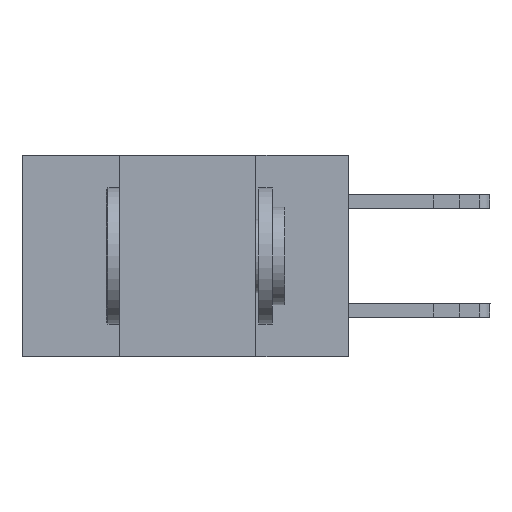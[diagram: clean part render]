
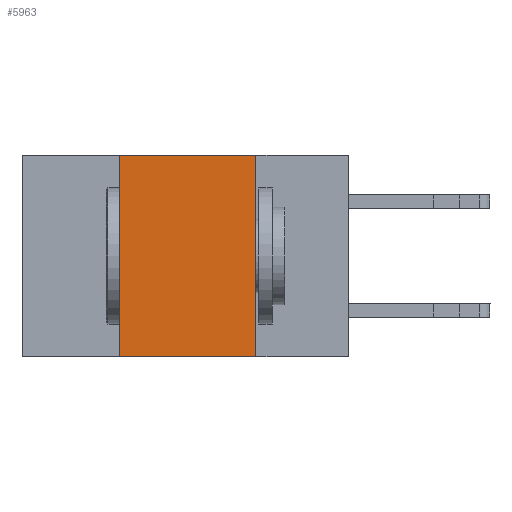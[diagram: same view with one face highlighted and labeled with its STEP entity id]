
A CAD part, left-side view. The second image highlights one B-rep face of the part: STEP entity #5963.
In plain terms, the highlighted planar face has unit normal (-1, 0, 0).
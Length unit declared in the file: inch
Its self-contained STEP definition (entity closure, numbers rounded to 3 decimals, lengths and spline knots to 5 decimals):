
#101 = ORIENTED_EDGE ( 'NONE', *, *, #4121, .F. ) ;
#929 = DIRECTION ( 'NONE',  ( 0., -1., 0. ) ) ;
#1136 = VERTEX_POINT ( 'NONE', #2300 ) ;
#1154 = VECTOR ( 'NONE', #8800, 39.37008 ) ;
#1475 = CARTESIAN_POINT ( 'NONE',  ( 0., 0.17, 0. ) ) ;
#1583 = LINE ( 'NONE', #4087, #10183 ) ;
#1917 = EDGE_CURVE ( 'NONE', #1136, #8242, #1583, .T. ) ;
#1934 = LINE ( 'NONE', #7120, #1154 ) ;
#2142 = DIRECTION ( 'NONE',  ( 0., 0., -1. ) ) ;
#2300 = CARTESIAN_POINT ( 'NONE',  ( 0., 0.42, -0.37 ) ) ;
#3206 = DIRECTION ( 'NONE',  ( 0., -1., 0. ) ) ;
#3469 = AXIS2_PLACEMENT_3D ( 'NONE', #3813, #5595, #2142 ) ;
#3813 = CARTESIAN_POINT ( 'NONE',  ( 0., 0.6, 0. ) ) ;
#3879 = PLANE ( 'NONE',  #3469 ) ;
#3974 = CARTESIAN_POINT ( 'NONE',  ( 0., 0.6, 0. ) ) ;
#4087 = CARTESIAN_POINT ( 'NONE',  ( 0., 0.42, -0.37 ) ) ;
#4121 = EDGE_CURVE ( 'NONE', #8177, #4962, #1934, .T. ) ;
#4219 = FACE_OUTER_BOUND ( 'NONE', #10107, .T. ) ;
#4271 = ORIENTED_EDGE ( 'NONE', *, *, #5785, .T. ) ;
#4962 = VERTEX_POINT ( 'NONE', #9652 ) ;
#5595 = DIRECTION ( 'NONE',  ( 1., 0., 0. ) ) ;
#5680 = EDGE_CURVE ( 'NONE', #8242, #8177, #10386, .T. ) ;
#5785 = EDGE_CURVE ( 'NONE', #1136, #4962, #7254, .T. ) ;
#5963 = ADVANCED_FACE ( 'NONE', ( #4219 ), #3879, .F. ) ;
#7120 = CARTESIAN_POINT ( 'NONE',  ( 0., 0.17, -0.37 ) ) ;
#7254 = LINE ( 'NONE', #7487, #10117 ) ;
#7487 = CARTESIAN_POINT ( 'NONE',  ( 0., 0.6, -0.37 ) ) ;
#8177 = VERTEX_POINT ( 'NONE', #1475 ) ;
#8242 = VERTEX_POINT ( 'NONE', #8365 ) ;
#8365 = CARTESIAN_POINT ( 'NONE',  ( 0., 0.42, 0. ) ) ;
#8800 = DIRECTION ( 'NONE',  ( 0., 0., -1. ) ) ;
#9614 = ORIENTED_EDGE ( 'NONE', *, *, #5680, .F. ) ;
#9652 = CARTESIAN_POINT ( 'NONE',  ( 0., 0.17, -0.37 ) ) ;
#10017 = DIRECTION ( 'NONE',  ( 0., 0., 1. ) ) ;
#10107 = EDGE_LOOP ( 'NONE', ( #101, #9614, #10415, #4271 ) ) ;
#10117 = VECTOR ( 'NONE', #929, 39.37008 ) ;
#10183 = VECTOR ( 'NONE', #10017, 39.37008 ) ;
#10386 = LINE ( 'NONE', #3974, #10654 ) ;
#10415 = ORIENTED_EDGE ( 'NONE', *, *, #1917, .F. ) ;
#10654 = VECTOR ( 'NONE', #3206, 39.37008 ) ;
